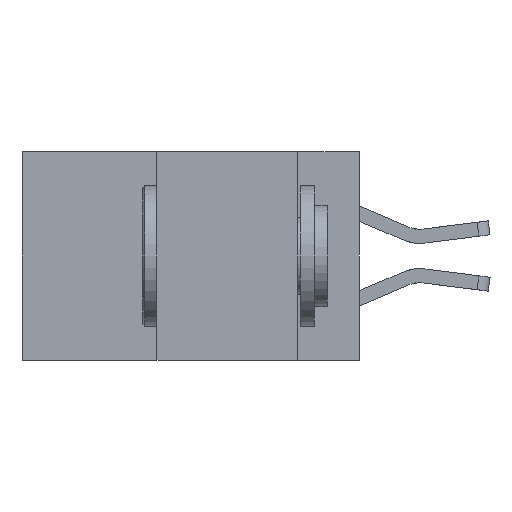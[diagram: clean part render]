
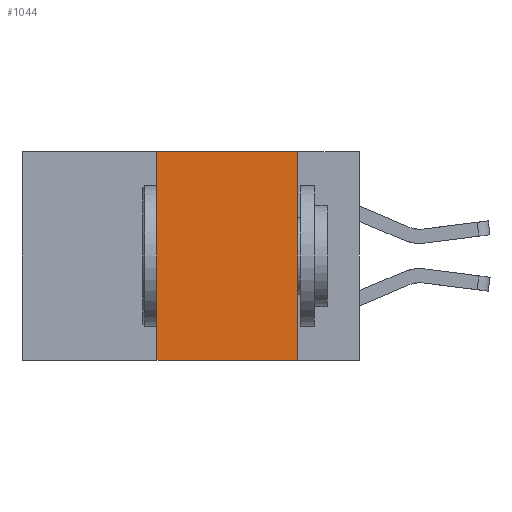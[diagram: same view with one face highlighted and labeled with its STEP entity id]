
A CAD part, left-side view. The second image highlights one B-rep face of the part: STEP entity #1044.
In plain terms, the highlighted planar face has unit normal (-1, 0, 0).
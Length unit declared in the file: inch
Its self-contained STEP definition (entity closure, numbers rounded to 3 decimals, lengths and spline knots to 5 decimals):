
#135 = VECTOR ( 'NONE', #678, 39.37008 ) ;
#319 = CARTESIAN_POINT ( 'NONE',  ( 0., 0.11, 0. ) ) ;
#678 = DIRECTION ( 'NONE',  ( 0., 0., 1. ) ) ;
#780 = DIRECTION ( 'NONE',  ( 0., -1., 0. ) ) ;
#1044 = ADVANCED_FACE ( 'NONE', ( #3684 ), #2201, .F. ) ;
#1143 = AXIS2_PLACEMENT_3D ( 'NONE', #7574, #6863, #4624 ) ;
#1154 = VECTOR ( 'NONE', #7016, 39.37008 ) ;
#1620 = ORIENTED_EDGE ( 'NONE', *, *, #9647, .F. ) ;
#2005 = VERTEX_POINT ( 'NONE', #3506 ) ;
#2201 = PLANE ( 'NONE',  #1143 ) ;
#2317 = EDGE_CURVE ( 'NONE', #2005, #5794, #2585, .T. ) ;
#2585 = LINE ( 'NONE', #6698, #135 ) ;
#3258 = LINE ( 'NONE', #9216, #1154 ) ;
#3506 = CARTESIAN_POINT ( 'NONE',  ( 0., 0.36, -0.37 ) ) ;
#3684 = FACE_OUTER_BOUND ( 'NONE', #7025, .T. ) ;
#3715 = ORIENTED_EDGE ( 'NONE', *, *, #2317, .F. ) ;
#4624 = DIRECTION ( 'NONE',  ( 0., 0., -1. ) ) ;
#5348 = LINE ( 'NONE', #6260, #5577 ) ;
#5418 = VERTEX_POINT ( 'NONE', #9418 ) ;
#5577 = VECTOR ( 'NONE', #780, 39.37008 ) ;
#5794 = VERTEX_POINT ( 'NONE', #7711 ) ;
#5976 = EDGE_CURVE ( 'NONE', #7050, #5418, #8277, .T. ) ;
#6260 = CARTESIAN_POINT ( 'NONE',  ( 0., 0.6, 0. ) ) ;
#6655 = CARTESIAN_POINT ( 'NONE',  ( 0., 0.11, 0. ) ) ;
#6698 = CARTESIAN_POINT ( 'NONE',  ( 0., 0.36, 0. ) ) ;
#6863 = DIRECTION ( 'NONE',  ( 1., 0., 0. ) ) ;
#6900 = DIRECTION ( 'NONE',  ( 0., 0., -1. ) ) ;
#7016 = DIRECTION ( 'NONE',  ( 0., -1., 0. ) ) ;
#7025 = EDGE_LOOP ( 'NONE', ( #9484, #1620, #3715, #7739 ) ) ;
#7050 = VERTEX_POINT ( 'NONE', #319 ) ;
#7574 = CARTESIAN_POINT ( 'NONE',  ( 0., 0.6, 0. ) ) ;
#7711 = CARTESIAN_POINT ( 'NONE',  ( 0., 0.36, 0. ) ) ;
#7739 = ORIENTED_EDGE ( 'NONE', *, *, #9640, .T. ) ;
#8277 = LINE ( 'NONE', #6655, #9977 ) ;
#9216 = CARTESIAN_POINT ( 'NONE',  ( 0., 0.6, -0.37 ) ) ;
#9418 = CARTESIAN_POINT ( 'NONE',  ( 0., 0.11, -0.37 ) ) ;
#9484 = ORIENTED_EDGE ( 'NONE', *, *, #5976, .F. ) ;
#9640 = EDGE_CURVE ( 'NONE', #2005, #5418, #3258, .T. ) ;
#9647 = EDGE_CURVE ( 'NONE', #5794, #7050, #5348, .T. ) ;
#9977 = VECTOR ( 'NONE', #6900, 39.37008 ) ;
